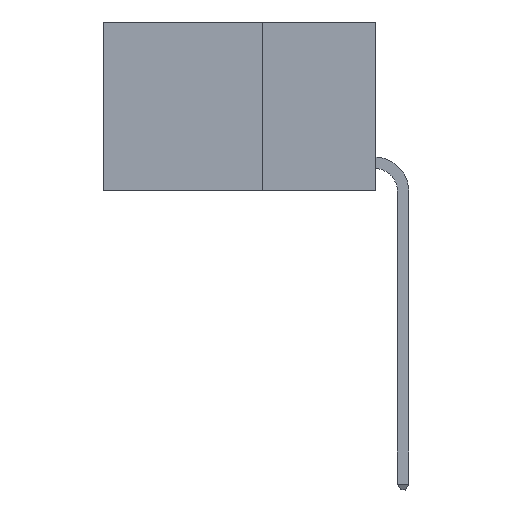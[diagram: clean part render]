
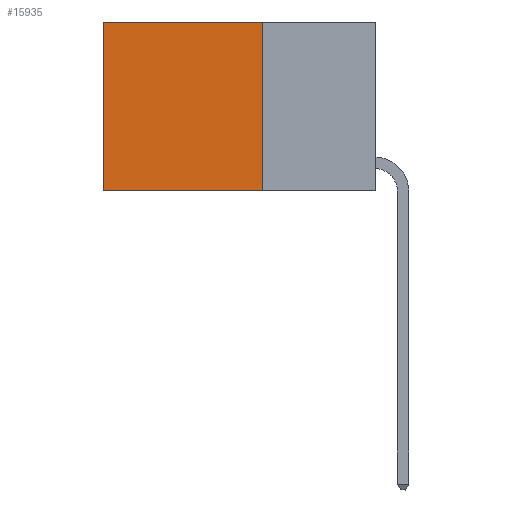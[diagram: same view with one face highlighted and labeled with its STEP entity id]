
A CAD part, left-side view. The second image highlights one B-rep face of the part: STEP entity #15935.
In plain terms, the highlighted planar face has unit normal (-1, 0, 0).
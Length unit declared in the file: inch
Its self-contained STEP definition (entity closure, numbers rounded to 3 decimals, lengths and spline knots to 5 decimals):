
#2043 = VECTOR ( 'NONE', #9739, 39.37008 ) ;
#2141 = VECTOR ( 'NONE', #7256, 39.37008 ) ;
#2539 = ORIENTED_EDGE ( 'NONE', *, *, #17561, .F. ) ;
#2939 = DIRECTION ( 'NONE',  ( 0., 1., 0. ) ) ;
#3523 = PLANE ( 'NONE',  #16402 ) ;
#4774 = CARTESIAN_POINT ( 'NONE',  ( 0.2625, 0.25, 0. ) ) ;
#5794 = EDGE_CURVE ( 'NONE', #13022, #23986, #6721, .T. ) ;
#5813 = VERTEX_POINT ( 'NONE', #9213 ) ;
#6195 = VERTEX_POINT ( 'NONE', #18220 ) ;
#6721 = LINE ( 'NONE', #18850, #2141 ) ;
#7256 = DIRECTION ( 'NONE',  ( 0., 0., -1. ) ) ;
#7464 = CARTESIAN_POINT ( 'NONE',  ( 0.2625, 0.25, 0. ) ) ;
#9213 = CARTESIAN_POINT ( 'NONE',  ( 0.2625, 0.6, -0.37 ) ) ;
#9739 = DIRECTION ( 'NONE',  ( 0., 0., -1. ) ) ;
#11365 = DIRECTION ( 'NONE',  ( 0., 0., -1. ) ) ;
#12659 = VECTOR ( 'NONE', #2939, 39.37008 ) ;
#12941 = CARTESIAN_POINT ( 'NONE',  ( 0.2625, 0.25, 0. ) ) ;
#13022 = VERTEX_POINT ( 'NONE', #12941 ) ;
#13666 = ORIENTED_EDGE ( 'NONE', *, *, #16888, .T. ) ;
#14210 = VECTOR ( 'NONE', #14454, 39.37008 ) ;
#14454 = DIRECTION ( 'NONE',  ( 0., 1., 0. ) ) ;
#15935 = ADVANCED_FACE ( 'NONE', ( #19999 ), #3523, .F. ) ;
#16298 = LINE ( 'NONE', #23277, #2043 ) ;
#16402 = AXIS2_PLACEMENT_3D ( 'NONE', #7464, #22955, #11365 ) ;
#16888 = EDGE_CURVE ( 'NONE', #13022, #6195, #19948, .T. ) ;
#17561 = EDGE_CURVE ( 'NONE', #23986, #5813, #23580, .T. ) ;
#18220 = CARTESIAN_POINT ( 'NONE',  ( 0.2625, 0.6, 0. ) ) ;
#18389 = CARTESIAN_POINT ( 'NONE',  ( 0.2625, 0.25, -0.37 ) ) ;
#18850 = CARTESIAN_POINT ( 'NONE',  ( 0.2625, 0.25, 0. ) ) ;
#19117 = ORIENTED_EDGE ( 'NONE', *, *, #21010, .T. ) ;
#19821 = CARTESIAN_POINT ( 'NONE',  ( 0.2625, 0.25, -0.37 ) ) ;
#19948 = LINE ( 'NONE', #4774, #14210 ) ;
#19999 = FACE_OUTER_BOUND ( 'NONE', #23462, .T. ) ;
#21010 = EDGE_CURVE ( 'NONE', #6195, #5813, #16298, .T. ) ;
#22648 = ORIENTED_EDGE ( 'NONE', *, *, #5794, .F. ) ;
#22955 = DIRECTION ( 'NONE',  ( 1., 0., 0. ) ) ;
#23277 = CARTESIAN_POINT ( 'NONE',  ( 0.2625, 0.6, 0. ) ) ;
#23462 = EDGE_LOOP ( 'NONE', ( #19117, #2539, #22648, #13666 ) ) ;
#23580 = LINE ( 'NONE', #18389, #12659 ) ;
#23986 = VERTEX_POINT ( 'NONE', #19821 ) ;
